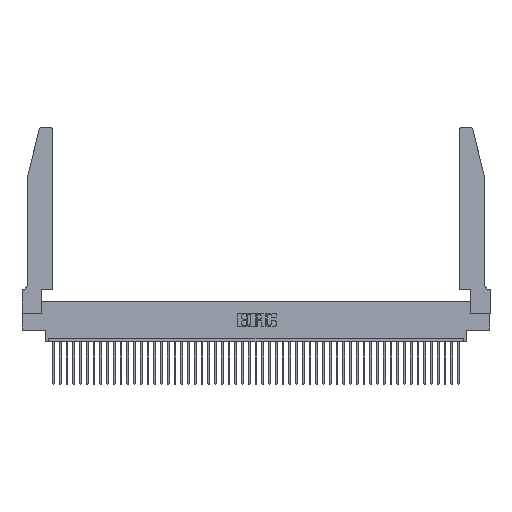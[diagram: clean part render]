
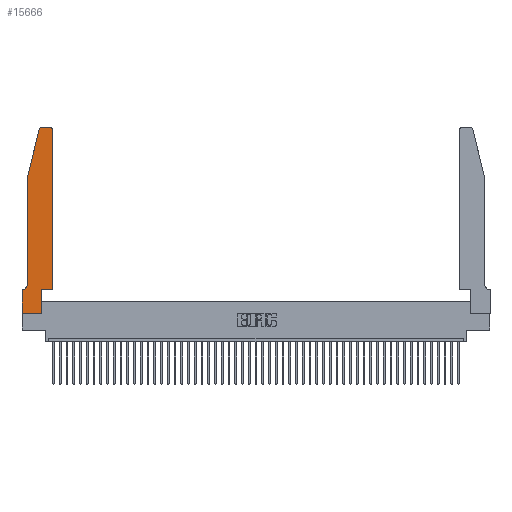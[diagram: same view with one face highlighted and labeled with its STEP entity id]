
A CAD part, top view. The second image highlights one B-rep face of the part: STEP entity #15666.
In plain terms, the highlighted planar face has unit normal (0, 0, 1).
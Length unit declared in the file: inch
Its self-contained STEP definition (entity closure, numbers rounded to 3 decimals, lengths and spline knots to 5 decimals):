
#150 = CARTESIAN_POINT ( 'NONE',  ( 0.4205, 2.75, 0.37 ) ) ;
#1268 = EDGE_CURVE ( 'NONE', #33766, #5998, #31722, .T. ) ;
#1403 = EDGE_CURVE ( 'NONE', #19699, #33755, #32300, .T. ) ;
#1886 = VECTOR ( 'NONE', #16215, 39.37008 ) ;
#2353 = EDGE_CURVE ( 'NONE', #36046, #33766, #20487, .T. ) ;
#2515 = VECTOR ( 'NONE', #12381, 39.37008 ) ;
#3177 = VERTEX_POINT ( 'NONE', #150 ) ;
#3489 = DIRECTION ( 'NONE',  ( 0., -1., 0. ) ) ;
#3559 = ORIENTED_EDGE ( 'NONE', *, *, #46431, .T. ) ;
#3984 = AXIS2_PLACEMENT_3D ( 'NONE', #34850, #9117, #38928 ) ;
#4824 = AXIS2_PLACEMENT_3D ( 'NONE', #14116, #39726, #17424 ) ;
#5998 = VERTEX_POINT ( 'NONE', #21242 ) ;
#6233 = LINE ( 'NONE', #25678, #12070 ) ;
#6246 = ORIENTED_EDGE ( 'NONE', *, *, #1403, .T. ) ;
#6541 = CIRCLE ( 'NONE', #4824, 0.03 ) ;
#7195 = EDGE_CURVE ( 'NONE', #34359, #24426, #22903, .T. ) ;
#8243 = CARTESIAN_POINT ( 'NONE',  ( 0.4505, 0.35, 0.37 ) ) ;
#9008 = CARTESIAN_POINT ( 'NONE',  ( 0.0755, 0.42, 0.37 ) ) ;
#9108 = ORIENTED_EDGE ( 'NONE', *, *, #39319, .T. ) ;
#9117 = DIRECTION ( 'NONE',  ( 0., 0., 1. ) ) ;
#9573 = VECTOR ( 'NONE', #20082, 39.37008 ) ;
#11339 = CARTESIAN_POINT ( 'NONE',  ( 0., 0., 0.37 ) ) ;
#12070 = VECTOR ( 'NONE', #40663, 39.37008 ) ;
#12381 = DIRECTION ( 'NONE',  ( 1., 0., 0. ) ) ;
#12481 = CARTESIAN_POINT ( 'NONE',  ( 0.0055, 0.42, 0.37 ) ) ;
#13033 = LINE ( 'NONE', #37951, #2515 ) ;
#13278 = VERTEX_POINT ( 'NONE', #23806 ) ;
#13313 = DIRECTION ( 'NONE',  ( -1., 0., 0. ) ) ;
#13352 = LINE ( 'NONE', #18636, #43046 ) ;
#13466 = CARTESIAN_POINT ( 'NONE',  ( 0.2865, 0.35, 0.37 ) ) ;
#14023 = CARTESIAN_POINT ( 'NONE',  ( 0.4505, 0.35, 0.37 ) ) ;
#14116 = CARTESIAN_POINT ( 'NONE',  ( 0.284, 2.72, 0.37 ) ) ;
#14133 = VECTOR ( 'NONE', #19005, 39.37008 ) ;
#15666 = ADVANCED_FACE ( 'NONE', ( #45832 ), #46214, .T. ) ;
#15947 = VERTEX_POINT ( 'NONE', #20740 ) ;
#16215 = DIRECTION ( 'NONE',  ( -0.239, -0.971, 0. ) ) ;
#16258 = DIRECTION ( 'NONE',  ( 0., 1., 0. ) ) ;
#17152 = CIRCLE ( 'NONE', #32395, 0.03 ) ;
#17424 = DIRECTION ( 'NONE',  ( 1., 0., 0. ) ) ;
#17570 = CARTESIAN_POINT ( 'NONE',  ( 0.2865, 0., 0.37 ) ) ;
#17901 = EDGE_CURVE ( 'NONE', #33983, #35313, #13033, .T. ) ;
#18636 = CARTESIAN_POINT ( 'NONE',  ( 0., 0., 0.37 ) ) ;
#19005 = DIRECTION ( 'NONE',  ( 1., 0., 0. ) ) ;
#19096 = ORIENTED_EDGE ( 'NONE', *, *, #7195, .T. ) ;
#19234 = ORIENTED_EDGE ( 'NONE', *, *, #17901, .T. ) ;
#19699 = VERTEX_POINT ( 'NONE', #31877 ) ;
#20082 = DIRECTION ( 'NONE',  ( -1., 0., 0. ) ) ;
#20286 = CARTESIAN_POINT ( 'NONE',  ( 0.0055, 0.35, 0.37 ) ) ;
#20487 = LINE ( 'NONE', #8243, #14133 ) ;
#20740 = CARTESIAN_POINT ( 'NONE',  ( 0.284, 2.75, 0.37 ) ) ;
#21202 = VECTOR ( 'NONE', #42339, 39.37008 ) ;
#21242 = CARTESIAN_POINT ( 'NONE',  ( 0.4505, 2.72, 0.37 ) ) ;
#22259 = ORIENTED_EDGE ( 'NONE', *, *, #2353, .T. ) ;
#22903 = CIRCLE ( 'NONE', #42890, 0.07 ) ;
#23326 = ORIENTED_EDGE ( 'NONE', *, *, #27619, .T. ) ;
#23377 = ORIENTED_EDGE ( 'NONE', *, *, #29847, .T. ) ;
#23506 = LINE ( 'NONE', #27564, #9573 ) ;
#23806 = CARTESIAN_POINT ( 'NONE',  ( 0., 0.35, 0.37 ) ) ;
#23998 = EDGE_CURVE ( 'NONE', #15947, #19699, #6541, .T. ) ;
#24426 = VERTEX_POINT ( 'NONE', #20286 ) ;
#24632 = CARTESIAN_POINT ( 'NONE',  ( 0.4205, 2.72, 0.37 ) ) ;
#24716 = ORIENTED_EDGE ( 'NONE', *, *, #34678, .T. ) ;
#25678 = CARTESIAN_POINT ( 'NONE',  ( 0.2605, 2.75, 0.37 ) ) ;
#26001 = DIRECTION ( 'NONE',  ( 0., -1., 0. ) ) ;
#27193 = CARTESIAN_POINT ( 'NONE',  ( 0.4505, 0.35, 0.37 ) ) ;
#27564 = CARTESIAN_POINT ( 'NONE',  ( 0.0755, 0.35, 0.37 ) ) ;
#27619 = EDGE_CURVE ( 'NONE', #3177, #15947, #6233, .T. ) ;
#29783 = EDGE_CURVE ( 'NONE', #24426, #13278, #23506, .T. ) ;
#29847 = EDGE_CURVE ( 'NONE', #35313, #36046, #41028, .T. ) ;
#30661 = ORIENTED_EDGE ( 'NONE', *, *, #1268, .T. ) ;
#31151 = ORIENTED_EDGE ( 'NONE', *, *, #29783, .T. ) ;
#31234 = DIRECTION ( 'NONE',  ( 0., 0., -1. ) ) ;
#31722 = LINE ( 'NONE', #27193, #21202 ) ;
#31764 = VECTOR ( 'NONE', #16258, 39.37008 ) ;
#31877 = CARTESIAN_POINT ( 'NONE',  ( 0.25487, 2.72718, 0.37 ) ) ;
#32300 = LINE ( 'NONE', #40511, #1886 ) ;
#32395 = AXIS2_PLACEMENT_3D ( 'NONE', #24632, #35578, #36227 ) ;
#32496 = EDGE_LOOP ( 'NONE', ( #23326, #43531, #6246, #24716, #19096, #31151, #3559, #19234, #23377, #22259, #30661, #9108 ) ) ;
#33755 = VERTEX_POINT ( 'NONE', #43815 ) ;
#33766 = VERTEX_POINT ( 'NONE', #14023 ) ;
#33983 = VERTEX_POINT ( 'NONE', #11339 ) ;
#34359 = VERTEX_POINT ( 'NONE', #9008 ) ;
#34678 = EDGE_CURVE ( 'NONE', #33755, #34359, #38028, .T. ) ;
#34850 = CARTESIAN_POINT ( 'NONE',  ( 0., 0.35, 0.37 ) ) ;
#35313 = VERTEX_POINT ( 'NONE', #17570 ) ;
#35578 = DIRECTION ( 'NONE',  ( 0., 0., 1. ) ) ;
#36046 = VERTEX_POINT ( 'NONE', #13466 ) ;
#36227 = DIRECTION ( 'NONE',  ( 1., 0., 0. ) ) ;
#37895 = CARTESIAN_POINT ( 'NONE',  ( 0.0755, 2., 0.37 ) ) ;
#37951 = CARTESIAN_POINT ( 'NONE',  ( 0., 0., 0.37 ) ) ;
#38028 = LINE ( 'NONE', #37895, #40325 ) ;
#38928 = DIRECTION ( 'NONE',  ( 1., 0., 0. ) ) ;
#39319 = EDGE_CURVE ( 'NONE', #5998, #3177, #17152, .T. ) ;
#39726 = DIRECTION ( 'NONE',  ( 0., 0., 1. ) ) ;
#40325 = VECTOR ( 'NONE', #26001, 39.37008 ) ;
#40511 = CARTESIAN_POINT ( 'NONE',  ( 0.0755, 2., 0.37 ) ) ;
#40663 = DIRECTION ( 'NONE',  ( -1., 0., 0. ) ) ;
#41028 = LINE ( 'NONE', #46206, #31764 ) ;
#42339 = DIRECTION ( 'NONE',  ( 0., 1., 0. ) ) ;
#42890 = AXIS2_PLACEMENT_3D ( 'NONE', #12481, #31234, #13313 ) ;
#43046 = VECTOR ( 'NONE', #3489, 39.37008 ) ;
#43531 = ORIENTED_EDGE ( 'NONE', *, *, #23998, .T. ) ;
#43815 = CARTESIAN_POINT ( 'NONE',  ( 0.0755, 2., 0.37 ) ) ;
#45832 = FACE_OUTER_BOUND ( 'NONE', #32496, .T. ) ;
#46206 = CARTESIAN_POINT ( 'NONE',  ( 0.2865, 0.35, 0.37 ) ) ;
#46214 = PLANE ( 'NONE',  #3984 ) ;
#46431 = EDGE_CURVE ( 'NONE', #13278, #33983, #13352, .T. ) ;
